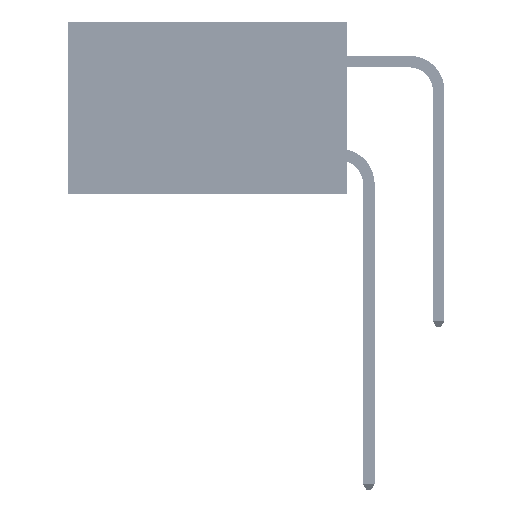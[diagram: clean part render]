
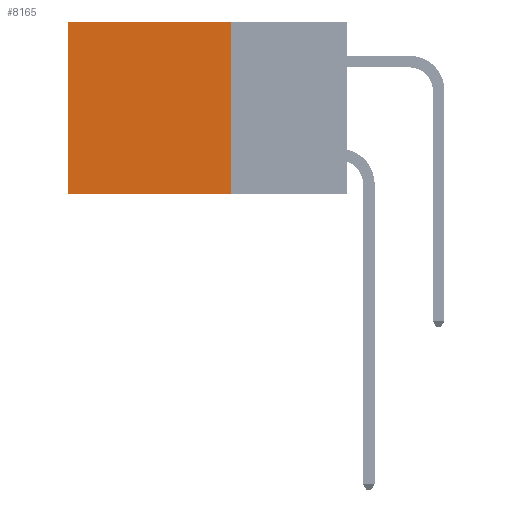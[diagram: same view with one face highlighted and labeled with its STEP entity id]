
A CAD part, left-side view. The second image highlights one B-rep face of the part: STEP entity #8165.
In plain terms, the highlighted planar face has unit normal (-1, 0, 0).
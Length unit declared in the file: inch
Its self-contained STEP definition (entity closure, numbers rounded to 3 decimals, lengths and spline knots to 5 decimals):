
#202 = ORIENTED_EDGE ( 'NONE', *, *, #14816, .T. ) ;
#3637 = CARTESIAN_POINT ( 'NONE',  ( 0.2875, 0.6, 0. ) ) ;
#4513 = VECTOR ( 'NONE', #23168, 39.37008 ) ;
#5511 = AXIS2_PLACEMENT_3D ( 'NONE', #37205, #17691, #33352 ) ;
#6782 = DIRECTION ( 'NONE',  ( 0., 0., -1. ) ) ;
#7522 = CARTESIAN_POINT ( 'NONE',  ( 0.2875, 0.25, 0. ) ) ;
#8165 = ADVANCED_FACE ( 'NONE', ( #41293 ), #21548, .F. ) ;
#9111 = EDGE_LOOP ( 'NONE', ( #202, #29866, #10755, #23881 ) ) ;
#10755 = ORIENTED_EDGE ( 'NONE', *, *, #50428, .F. ) ;
#11163 = LINE ( 'NONE', #19126, #49453 ) ;
#12647 = CARTESIAN_POINT ( 'NONE',  ( 0.2875, 0.25, 0. ) ) ;
#14816 = EDGE_CURVE ( 'NONE', #38051, #18010, #45755, .T. ) ;
#16881 = VECTOR ( 'NONE', #31264, 39.37008 ) ;
#17691 = DIRECTION ( 'NONE',  ( 1., 0., 0. ) ) ;
#18010 = VERTEX_POINT ( 'NONE', #31376 ) ;
#19126 = CARTESIAN_POINT ( 'NONE',  ( 0.2875, 0.25, -0.37 ) ) ;
#21548 = PLANE ( 'NONE',  #5511 ) ;
#22881 = EDGE_CURVE ( 'NONE', #41354, #38051, #50356, .T. ) ;
#23168 = DIRECTION ( 'NONE',  ( 0., 1., 0. ) ) ;
#23881 = ORIENTED_EDGE ( 'NONE', *, *, #22881, .T. ) ;
#25171 = CARTESIAN_POINT ( 'NONE',  ( 0.2875, 0.25, -0.37 ) ) ;
#29866 = ORIENTED_EDGE ( 'NONE', *, *, #35580, .F. ) ;
#31264 = DIRECTION ( 'NONE',  ( 0., 0., -1. ) ) ;
#31376 = CARTESIAN_POINT ( 'NONE',  ( 0.2875, 0.6, -0.37 ) ) ;
#33203 = CARTESIAN_POINT ( 'NONE',  ( 0.2875, 0.6, 0. ) ) ;
#33352 = DIRECTION ( 'NONE',  ( 0., 0., -1. ) ) ;
#35580 = EDGE_CURVE ( 'NONE', #40265, #18010, #11163, .T. ) ;
#36108 = CARTESIAN_POINT ( 'NONE',  ( 0.2875, 0.25, 0. ) ) ;
#37205 = CARTESIAN_POINT ( 'NONE',  ( 0.2875, 0.25, 0. ) ) ;
#38051 = VERTEX_POINT ( 'NONE', #3637 ) ;
#38363 = DIRECTION ( 'NONE',  ( 0., 1., 0. ) ) ;
#38951 = LINE ( 'NONE', #36108, #16881 ) ;
#40265 = VERTEX_POINT ( 'NONE', #25171 ) ;
#41293 = FACE_OUTER_BOUND ( 'NONE', #9111, .T. ) ;
#41354 = VERTEX_POINT ( 'NONE', #12647 ) ;
#45755 = LINE ( 'NONE', #33203, #46810 ) ;
#46810 = VECTOR ( 'NONE', #6782, 39.37008 ) ;
#49453 = VECTOR ( 'NONE', #38363, 39.37008 ) ;
#50356 = LINE ( 'NONE', #7522, #4513 ) ;
#50428 = EDGE_CURVE ( 'NONE', #41354, #40265, #38951, .T. ) ;
